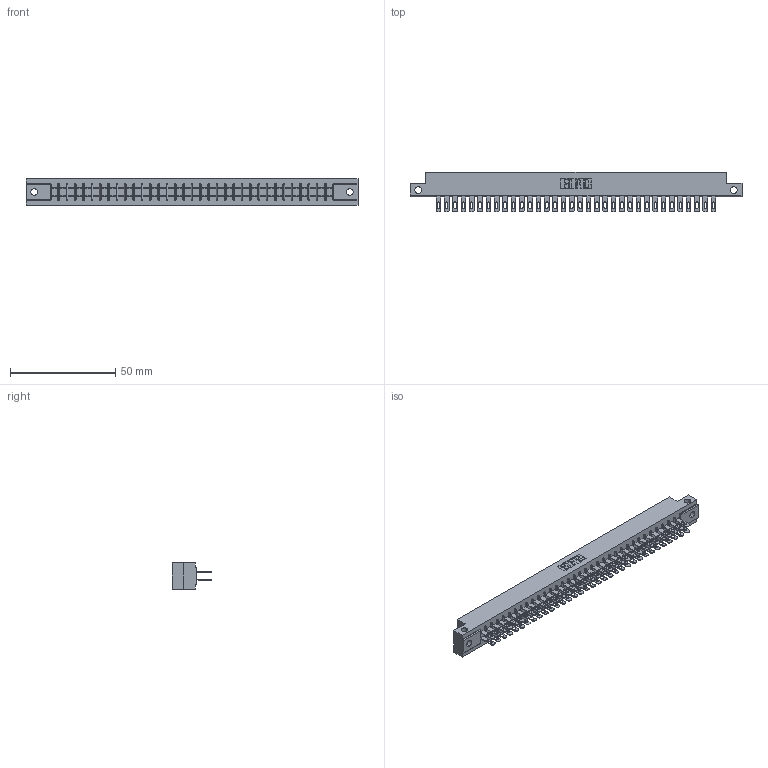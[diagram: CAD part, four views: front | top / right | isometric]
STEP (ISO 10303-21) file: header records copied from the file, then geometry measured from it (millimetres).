
FILE_DESCRIPTION (( 'STEP AP203' ), '1' );
FILE_NAME ('315-068-500-212.STEP', '2020-09-20T03:44:03', ( '' ), ( '' ), 'SwSTEP 2.0', 'SolidWorks 2020', '' );
FILE_SCHEMA (( 'CONFIG_CONTROL_DESIGN' ));
Length unit declared in the file: inch
Products named in the file (3): 305-290-001_500; 305 Part_.128 Dia; 315-068-500-212
Assembly tree (69 placements, depth 2):
  315-068-500-212
    305 Part_.128 Dia
    305-290-001_500  x68
Bounding box: 157.73 x 18.85 x 12.7 mm (x, y, z)
Volume: 16418.6 mm3; surface area: 22109.6 mm2
Topology: 69 solids, 69 shells, 3528 faces, 10110 edges, 6552 vertices
Faces by surface type: plane 1972, cylinder 1420, sphere 136
Entity records: 38215 total; most frequent: CARTESIAN_POINT 6372, ORIENTED_EDGE 6280, DIRECTION 6112, EDGE_CURVE 3140, LINE 2512, VECTOR 2512, VERTEX_POINT 1996, AXIS2_PLACEMENT_3D 1800
